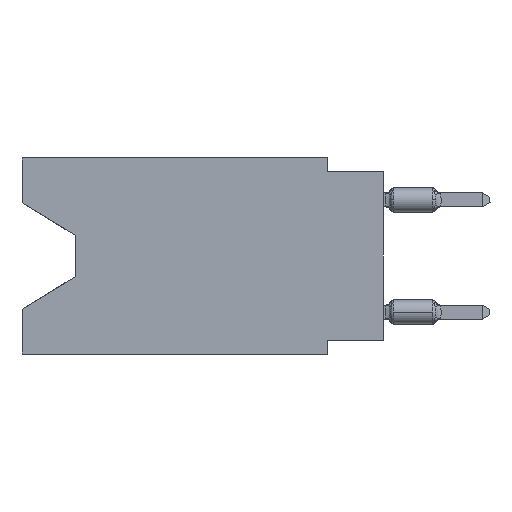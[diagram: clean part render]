
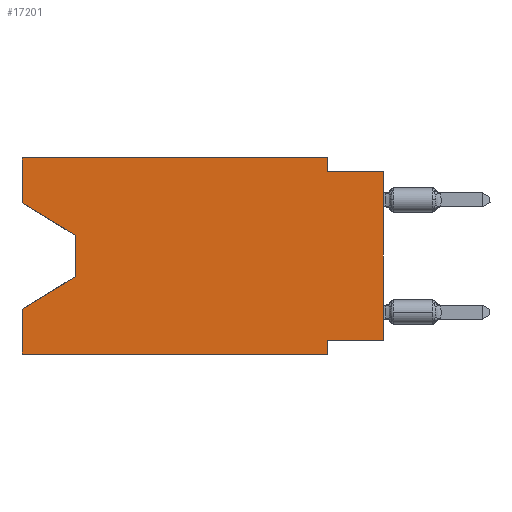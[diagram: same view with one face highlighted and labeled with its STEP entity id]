
A CAD part, left-side view. The second image highlights one B-rep face of the part: STEP entity #17201.
In plain terms, the highlighted planar face has unit normal (-1, 0, 0).
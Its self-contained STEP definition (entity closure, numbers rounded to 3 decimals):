
#294 = VERTEX_POINT ( 'NONE', #20815 ) ;
#448 = VECTOR ( 'NONE', #21200, 1000. ) ;
#518 = DIRECTION ( 'NONE',  ( 0., 0., -1. ) ) ;
#666 = VERTEX_POINT ( 'NONE', #11774 ) ;
#814 = VECTOR ( 'NONE', #9275, 1000. ) ;
#852 = EDGE_LOOP ( 'NONE', ( #2136, #16358, #19590, #6940, #16796, #9585, #6035, #20702, #8982, #7486, #7206, #21395 ) ) ;
#1979 = VERTEX_POINT ( 'NONE', #13562 ) ;
#2049 = LINE ( 'NONE', #9501, #3379 ) ;
#2136 = ORIENTED_EDGE ( 'NONE', *, *, #17802, .T. ) ;
#2168 = CARTESIAN_POINT ( 'NONE',  ( 0., 2.54, -8.89 ) ) ;
#2680 = LINE ( 'NONE', #15070, #7982 ) ;
#2790 = EDGE_CURVE ( 'NONE', #12158, #666, #5412, .T. ) ;
#3084 = VECTOR ( 'NONE', #518, 1000. ) ;
#3095 = CARTESIAN_POINT ( 'NONE',  ( 0., 16.383, -2.038 ) ) ;
#3140 = CARTESIAN_POINT ( 'NONE',  ( 0., 13.97, -5.385 ) ) ;
#3294 = EDGE_CURVE ( 'NONE', #294, #18171, #18001, .T. ) ;
#3379 = VECTOR ( 'NONE', #7642, 1000. ) ;
#3806 = EDGE_CURVE ( 'NONE', #15764, #5786, #14803, .T. ) ;
#4192 = CARTESIAN_POINT ( 'NONE',  ( 0., 2.54, -8.89 ) ) ;
#4224 = DIRECTION ( 'NONE',  ( 1., 0., 0. ) ) ;
#4236 = DIRECTION ( 'NONE',  ( 0., 0., 1. ) ) ;
#4673 = VERTEX_POINT ( 'NONE', #3140 ) ;
#4792 = VERTEX_POINT ( 'NONE', #23113 ) ;
#5122 = VERTEX_POINT ( 'NONE', #17121 ) ;
#5243 = VECTOR ( 'NONE', #5525, 1000. ) ;
#5267 = VECTOR ( 'NONE', #22935, 1000. ) ;
#5412 = LINE ( 'NONE', #14637, #17607 ) ;
#5525 = DIRECTION ( 'NONE',  ( 0., 1., 0. ) ) ;
#5704 = AXIS2_PLACEMENT_3D ( 'NONE', #16608, #4224, #14838 ) ;
#5733 = FACE_OUTER_BOUND ( 'NONE', #852, .T. ) ;
#5786 = VERTEX_POINT ( 'NONE', #4192 ) ;
#6035 = ORIENTED_EDGE ( 'NONE', *, *, #22315, .F. ) ;
#6749 = LINE ( 'NONE', #16952, #20240 ) ;
#6940 = ORIENTED_EDGE ( 'NONE', *, *, #3294, .F. ) ;
#7206 = ORIENTED_EDGE ( 'NONE', *, *, #22636, .F. ) ;
#7314 = CARTESIAN_POINT ( 'NONE',  ( 0., 2.54, -8.255 ) ) ;
#7486 = ORIENTED_EDGE ( 'NONE', *, *, #12510, .F. ) ;
#7634 = CARTESIAN_POINT ( 'NONE',  ( 0., 13.97, -3.505 ) ) ;
#7642 = DIRECTION ( 'NONE',  ( 0., 0., -1. ) ) ;
#7982 = VECTOR ( 'NONE', #18568, 1000. ) ;
#8017 = DIRECTION ( 'NONE',  ( 0., 0., 1. ) ) ;
#8270 = DIRECTION ( 'NONE',  ( 0., 0.855, -0.519 ) ) ;
#8841 = EDGE_CURVE ( 'NONE', #14747, #4673, #16541, .T. ) ;
#8982 = ORIENTED_EDGE ( 'NONE', *, *, #2790, .F. ) ;
#9195 = CARTESIAN_POINT ( 'NONE',  ( 0., 16.383, 0. ) ) ;
#9275 = DIRECTION ( 'NONE',  ( 0., 0., -1. ) ) ;
#9501 = CARTESIAN_POINT ( 'NONE',  ( 0., 2.54, 0. ) ) ;
#9585 = ORIENTED_EDGE ( 'NONE', *, *, #3806, .F. ) ;
#9688 = VECTOR ( 'NONE', #8017, 1000. ) ;
#10384 = LINE ( 'NONE', #22686, #5267 ) ;
#10535 = CARTESIAN_POINT ( 'NONE',  ( 0., 13.97, -3.505 ) ) ;
#10762 = LINE ( 'NONE', #19684, #5243 ) ;
#11774 = CARTESIAN_POINT ( 'NONE',  ( 0., 0., -0.635 ) ) ;
#11838 = LINE ( 'NONE', #3095, #448 ) ;
#12158 = VERTEX_POINT ( 'NONE', #15627 ) ;
#12510 = EDGE_CURVE ( 'NONE', #5122, #12158, #2049, .T. ) ;
#12992 = CARTESIAN_POINT ( 'NONE',  ( 0., 16.383, 0. ) ) ;
#13562 = CARTESIAN_POINT ( 'NONE',  ( 0., 16.383, -2.038 ) ) ;
#14637 = CARTESIAN_POINT ( 'NONE',  ( 0., 0., -0.635 ) ) ;
#14747 = VERTEX_POINT ( 'NONE', #10535 ) ;
#14803 = LINE ( 'NONE', #2168, #814 ) ;
#14838 = DIRECTION ( 'NONE',  ( 0., 0., -1. ) ) ;
#14847 = CARTESIAN_POINT ( 'NONE',  ( 0., 16.383, 0. ) ) ;
#15070 = CARTESIAN_POINT ( 'NONE',  ( 0., 16.383, -8.89 ) ) ;
#15079 = PLANE ( 'NONE',  #5704 ) ;
#15627 = CARTESIAN_POINT ( 'NONE',  ( 0., 2.54, -0.635 ) ) ;
#15764 = VERTEX_POINT ( 'NONE', #7314 ) ;
#16162 = VERTEX_POINT ( 'NONE', #12992 ) ;
#16167 = DIRECTION ( 'NONE',  ( 0., -1., 0. ) ) ;
#16358 = ORIENTED_EDGE ( 'NONE', *, *, #8841, .T. ) ;
#16541 = LINE ( 'NONE', #7634, #3084 ) ;
#16608 = CARTESIAN_POINT ( 'NONE',  ( 0., 16.383, 0. ) ) ;
#16677 = EDGE_CURVE ( 'NONE', #294, #5786, #2680, .T. ) ;
#16796 = ORIENTED_EDGE ( 'NONE', *, *, #16677, .T. ) ;
#16952 = CARTESIAN_POINT ( 'NONE',  ( 0., 13.97, -5.385 ) ) ;
#17121 = CARTESIAN_POINT ( 'NONE',  ( 0., 2.54, 0. ) ) ;
#17201 = ADVANCED_FACE ( 'NONE', ( #5733 ), #15079, .F. ) ;
#17362 = EDGE_CURVE ( 'NONE', #4673, #18171, #6749, .T. ) ;
#17607 = VECTOR ( 'NONE', #16167, 1000. ) ;
#17802 = EDGE_CURVE ( 'NONE', #1979, #14747, #11838, .T. ) ;
#18001 = LINE ( 'NONE', #9195, #22467 ) ;
#18171 = VERTEX_POINT ( 'NONE', #21067 ) ;
#18568 = DIRECTION ( 'NONE',  ( 0., -1., 0. ) ) ;
#18794 = LINE ( 'NONE', #22410, #9688 ) ;
#18985 = EDGE_CURVE ( 'NONE', #4792, #666, #18794, .T. ) ;
#19590 = ORIENTED_EDGE ( 'NONE', *, *, #17362, .T. ) ;
#19684 = CARTESIAN_POINT ( 'NONE',  ( 0., 0., -8.255 ) ) ;
#19823 = EDGE_CURVE ( 'NONE', #1979, #16162, #20360, .T. ) ;
#20240 = VECTOR ( 'NONE', #8270, 1000. ) ;
#20360 = LINE ( 'NONE', #14847, #21300 ) ;
#20702 = ORIENTED_EDGE ( 'NONE', *, *, #18985, .T. ) ;
#20815 = CARTESIAN_POINT ( 'NONE',  ( 0., 16.383, -8.89 ) ) ;
#21067 = CARTESIAN_POINT ( 'NONE',  ( 0., 16.383, -6.852 ) ) ;
#21200 = DIRECTION ( 'NONE',  ( 0., -0.855, -0.519 ) ) ;
#21268 = DIRECTION ( 'NONE',  ( 0., 0., 1. ) ) ;
#21300 = VECTOR ( 'NONE', #4236, 1000. ) ;
#21395 = ORIENTED_EDGE ( 'NONE', *, *, #19823, .F. ) ;
#22315 = EDGE_CURVE ( 'NONE', #4792, #15764, #10762, .T. ) ;
#22410 = CARTESIAN_POINT ( 'NONE',  ( 0., 0., 0. ) ) ;
#22467 = VECTOR ( 'NONE', #21268, 1000. ) ;
#22636 = EDGE_CURVE ( 'NONE', #16162, #5122, #10384, .T. ) ;
#22686 = CARTESIAN_POINT ( 'NONE',  ( 0., 16.383, 0. ) ) ;
#22935 = DIRECTION ( 'NONE',  ( 0., -1., 0. ) ) ;
#23113 = CARTESIAN_POINT ( 'NONE',  ( 0., 0., -8.255 ) ) ;
